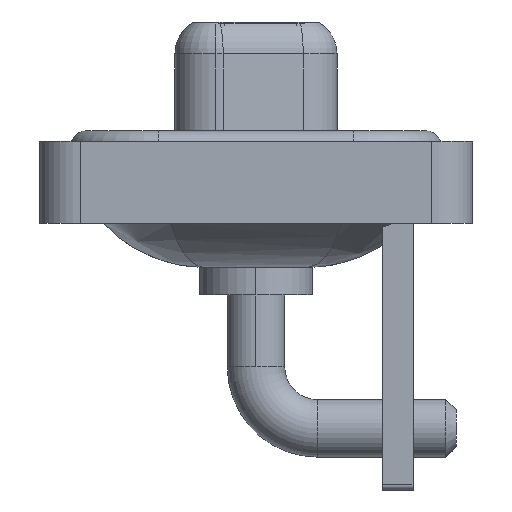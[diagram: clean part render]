
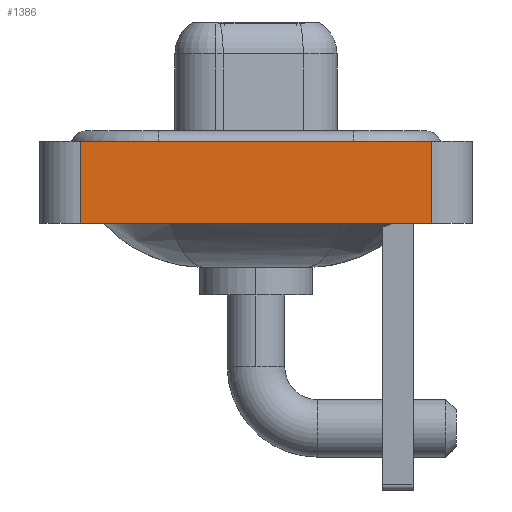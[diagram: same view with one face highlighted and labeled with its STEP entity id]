
A CAD part, left-side view. The second image highlights one B-rep face of the part: STEP entity #1386.
In plain terms, the highlighted planar face has unit normal (-1, 0, 0).
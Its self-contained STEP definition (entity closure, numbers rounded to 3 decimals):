
#247 = CARTESIAN_POINT ( 'NONE',  ( -7.3, 8.55, -3.6 ) ) ;
#1001 = CARTESIAN_POINT ( 'NONE',  ( -7.3, 8.55, -3.6 ) ) ;
#1386 = ADVANCED_FACE ( 'NONE', ( #10481 ), #5568, .T. ) ;
#2217 = EDGE_CURVE ( 'NONE', #7912, #4629, #7516, .T. ) ;
#2417 = LINE ( 'NONE', #10540, #15378 ) ;
#2571 = DIRECTION ( 'NONE',  ( 0., -1., 0. ) ) ;
#2577 = CARTESIAN_POINT ( 'NONE',  ( -7.3, -8.55, -3.6 ) ) ;
#3008 = ORIENTED_EDGE ( 'NONE', *, *, #12452, .T. ) ;
#3351 = ORIENTED_EDGE ( 'NONE', *, *, #5866, .F. ) ;
#4357 = ORIENTED_EDGE ( 'NONE', *, *, #11422, .T. ) ;
#4629 = VERTEX_POINT ( 'NONE', #6923 ) ;
#4691 = CARTESIAN_POINT ( 'NONE',  ( -7.3, -8.55, 0.4 ) ) ;
#5116 = DIRECTION ( 'NONE',  ( 0., 0., 1. ) ) ;
#5568 = PLANE ( 'NONE',  #14181 ) ;
#5866 = EDGE_CURVE ( 'NONE', #4629, #6326, #2417, .T. ) ;
#5976 = LINE ( 'NONE', #7281, #7530 ) ;
#6326 = VERTEX_POINT ( 'NONE', #4691 ) ;
#6923 = CARTESIAN_POINT ( 'NONE',  ( -7.3, 8.55, 0.4 ) ) ;
#7281 = CARTESIAN_POINT ( 'NONE',  ( -7.3, -8.55, -3.6 ) ) ;
#7516 = LINE ( 'NONE', #1001, #8157 ) ;
#7530 = VECTOR ( 'NONE', #16514, 1000. ) ;
#7747 = VERTEX_POINT ( 'NONE', #2577 ) ;
#7912 = VERTEX_POINT ( 'NONE', #247 ) ;
#8157 = VECTOR ( 'NONE', #5116, 1000. ) ;
#9073 = EDGE_LOOP ( 'NONE', ( #4357, #3351, #11910, #3008 ) ) ;
#10017 = VECTOR ( 'NONE', #2571, 1000. ) ;
#10268 = CARTESIAN_POINT ( 'NONE',  ( -7.3, -8.55, -3.6 ) ) ;
#10287 = DIRECTION ( 'NONE',  ( 0., -1., 0. ) ) ;
#10394 = CARTESIAN_POINT ( 'NONE',  ( -7.3, -8.55, -3.6 ) ) ;
#10481 = FACE_OUTER_BOUND ( 'NONE', #9073, .T. ) ;
#10540 = CARTESIAN_POINT ( 'NONE',  ( -7.3, -8.55, 0.4 ) ) ;
#10597 = LINE ( 'NONE', #10268, #10017 ) ;
#11422 = EDGE_CURVE ( 'NONE', #7747, #6326, #5976, .T. ) ;
#11910 = ORIENTED_EDGE ( 'NONE', *, *, #2217, .F. ) ;
#12452 = EDGE_CURVE ( 'NONE', #7912, #7747, #10597, .T. ) ;
#13347 = DIRECTION ( 'NONE',  ( -1., 0., 0. ) ) ;
#14181 = AXIS2_PLACEMENT_3D ( 'NONE', #10394, #13347, #16007 ) ;
#15378 = VECTOR ( 'NONE', #10287, 1000. ) ;
#16007 = DIRECTION ( 'NONE',  ( 0., 0., 1. ) ) ;
#16514 = DIRECTION ( 'NONE',  ( 0., 0., 1. ) ) ;
